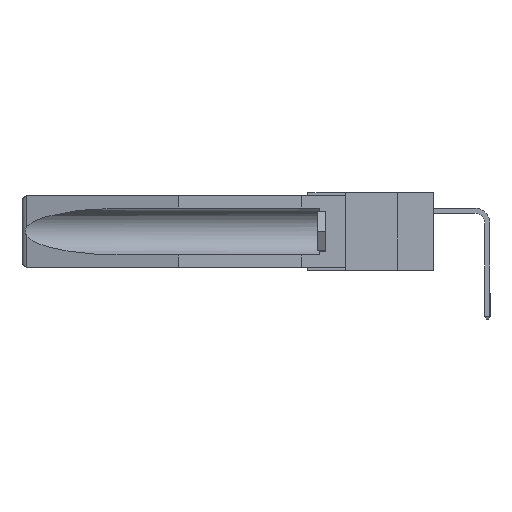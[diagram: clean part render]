
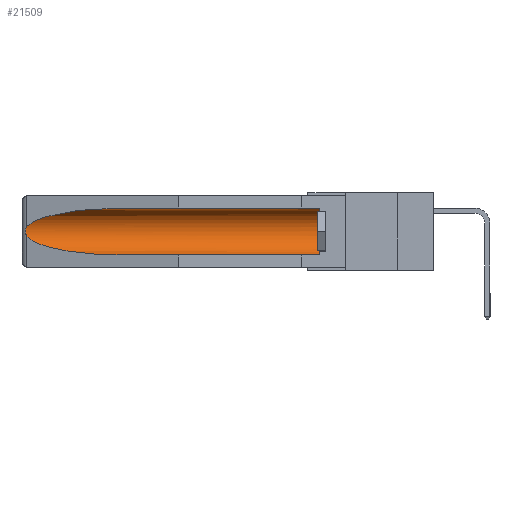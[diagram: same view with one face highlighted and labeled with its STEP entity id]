
A CAD part, left-side view. The second image highlights one B-rep face of the part: STEP entity #21509.
In plain terms, the highlighted cylindrical face has radius 2.857 mm (diameter 5.715 mm), a partial arc.
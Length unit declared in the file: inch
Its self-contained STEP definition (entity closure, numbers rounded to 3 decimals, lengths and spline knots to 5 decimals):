
#577 = CARTESIAN_POINT ( 'NONE',  ( 0.155, 0.126, -0.059 ) ) ;
#893 = DIRECTION ( 'NONE',  ( 0., -1., 0. ) ) ;
#1407 = VECTOR ( 'NONE', #24017, 39.37008 ) ;
#2414 = CARTESIAN_POINT ( 'NONE',  ( 0.26537, 1.52718, -0.14972 ) ) ;
#2586 = CYLINDRICAL_SURFACE ( 'NONE', #2621, 0.1125 ) ;
#2621 = AXIS2_PLACEMENT_3D ( 'NONE', #10202, #10101, #19785 ) ;
#2776 = ORIENTED_EDGE ( 'NONE', *, *, #7997, .T. ) ;
#2848 = CARTESIAN_POINT ( 'NONE',  ( 0.2673, 1.5327, -0.16383 ) ) ;
#3377 = FACE_OUTER_BOUND ( 'NONE', #18006, .T. ) ;
#3425 = CARTESIAN_POINT ( 'NONE',  ( 0.155, 1.07973, -0.059 ) ) ;
#3851 = EDGE_CURVE ( 'NONE', #27591, #8074, #8372, .T. ) ;
#4380 =( BOUNDED_CURVE ( )  B_SPLINE_CURVE ( 3, ( #20080, #9997, #12568, #12456 ),
 .UNSPECIFIED., .F., .F. ) 
 B_SPLINE_CURVE_WITH_KNOTS ( ( 4, 4 ),
 ( 0.1948, 1.5708 ),
 .UNSPECIFIED. ) 
 CURVE ( )  GEOMETRIC_REPRESENTATION_ITEM ( )  RATIONAL_B_SPLINE_CURVE ( ( 1., 0.848, 0.848, 1. ) ) 
 REPRESENTATION_ITEM ( '' )  );
#4825 = VERTEX_POINT ( 'NONE', #29679 ) ;
#4939 = CARTESIAN_POINT ( 'NONE',  ( 0.2675, 1.53308, -0.16763 ) ) ;
#5349 = CARTESIAN_POINT ( 'NONE',  ( 0.26654, 1.53092, -0.15636 ) ) ;
#5890 = DIRECTION ( 'NONE',  ( 0., 0., 1. ) ) ;
#6041 = CARTESIAN_POINT ( 'NONE',  ( 0.155, 0.126, -0.284 ) ) ;
#6759 = B_SPLINE_CURVE_WITH_KNOTS ( 'NONE', 3,
 ( #2414, #20089, #5349, #2848, #4939, #22578, #27215, #12468, #12373, #25037 ),
 .UNSPECIFIED., .F., .F.,
 ( 4, 2, 2, 2, 4 ),
 ( 0., 0.00029, 0.00058, 0.00087, 0.00117 ),
 .UNSPECIFIED. ) ;
#7787 = CARTESIAN_POINT ( 'NONE',  ( 0.26537, 1.52718, -0.19328 ) ) ;
#7997 = EDGE_CURVE ( 'NONE', #20278, #27591, #26233, .T. ) ;
#8074 = VERTEX_POINT ( 'NONE', #3425 ) ;
#8372 = LINE ( 'NONE', #26390, #1407 ) ;
#8554 =( BOUNDED_CURVE ( )  B_SPLINE_CURVE ( 3, ( #27789, #20243, #15435, #24977 ),
 .UNSPECIFIED., .F., .F. ) 
 B_SPLINE_CURVE_WITH_KNOTS ( ( 4, 4 ),
 ( 4.71239, 6.08839 ),
 .UNSPECIFIED. ) 
 CURVE ( )  GEOMETRIC_REPRESENTATION_ITEM ( )  RATIONAL_B_SPLINE_CURVE ( ( 1., 0.848, 0.848, 1. ) ) 
 REPRESENTATION_ITEM ( '' )  );
#8828 = VECTOR ( 'NONE', #14653, 39.37008 ) ;
#9297 = EDGE_CURVE ( 'NONE', #20278, #16588, #30841, .T. ) ;
#9997 = CARTESIAN_POINT ( 'NONE',  ( 0.25451, 1.48313, -0.24835 ) ) ;
#10101 = DIRECTION ( 'NONE',  ( 0., 1., 0. ) ) ;
#10202 = CARTESIAN_POINT ( 'NONE',  ( 0.155, -0.30754, -0.1715 ) ) ;
#10819 = EDGE_CURVE ( 'NONE', #8074, #4825, #8554, .T. ) ;
#11941 = EDGE_CURVE ( 'NONE', #15823, #16588, #4380, .T. ) ;
#12373 = CARTESIAN_POINT ( 'NONE',  ( 0.26597, 1.5296, -0.19026 ) ) ;
#12456 = CARTESIAN_POINT ( 'NONE',  ( 0.155, 1.07973, -0.284 ) ) ;
#12468 = CARTESIAN_POINT ( 'NONE',  ( 0.26655, 1.53094, -0.18657 ) ) ;
#12568 = CARTESIAN_POINT ( 'NONE',  ( 0.21114, 1.30732, -0.284 ) ) ;
#13247 = CARTESIAN_POINT ( 'NONE',  ( 0.155, 0.126, -0.1715 ) ) ;
#14653 = DIRECTION ( 'NONE',  ( 0., 1., 0. ) ) ;
#15435 = CARTESIAN_POINT ( 'NONE',  ( 0.25451, 1.48313, -0.09465 ) ) ;
#15823 = VERTEX_POINT ( 'NONE', #7787 ) ;
#16588 = VERTEX_POINT ( 'NONE', #21506 ) ;
#17845 = ORIENTED_EDGE ( 'NONE', *, *, #3851, .T. ) ;
#18006 = EDGE_LOOP ( 'NONE', ( #25649, #25445, #29173, #28825, #2776, #17845 ) ) ;
#19785 = DIRECTION ( 'NONE',  ( 0., 0., 1. ) ) ;
#20080 = CARTESIAN_POINT ( 'NONE',  ( 0.26537, 1.52718, -0.19328 ) ) ;
#20089 = CARTESIAN_POINT ( 'NONE',  ( 0.26597, 1.52961, -0.15275 ) ) ;
#20243 = CARTESIAN_POINT ( 'NONE',  ( 0.21114, 1.30732, -0.059 ) ) ;
#20278 = VERTEX_POINT ( 'NONE', #6041 ) ;
#21506 = CARTESIAN_POINT ( 'NONE',  ( 0.155, 1.07973, -0.284 ) ) ;
#21509 = ADVANCED_FACE ( 'NONE', ( #3377 ), #2586, .F. ) ;
#22139 = CARTESIAN_POINT ( 'NONE',  ( 0.155, -0.30754, -0.284 ) ) ;
#22502 = EDGE_CURVE ( 'NONE', #4825, #15823, #6759, .T. ) ;
#22578 = CARTESIAN_POINT ( 'NONE',  ( 0.2675, 1.53308, -0.17534 ) ) ;
#24017 = DIRECTION ( 'NONE',  ( 0., 1., 0. ) ) ;
#24977 = CARTESIAN_POINT ( 'NONE',  ( 0.26537, 1.52718, -0.14972 ) ) ;
#25037 = CARTESIAN_POINT ( 'NONE',  ( 0.26537, 1.52718, -0.19328 ) ) ;
#25445 = ORIENTED_EDGE ( 'NONE', *, *, #22502, .T. ) ;
#25649 = ORIENTED_EDGE ( 'NONE', *, *, #10819, .T. ) ;
#26233 = CIRCLE ( 'NONE', #26742, 0.1125 ) ;
#26390 = CARTESIAN_POINT ( 'NONE',  ( 0.155, -0.30754, -0.059 ) ) ;
#26742 = AXIS2_PLACEMENT_3D ( 'NONE', #13247, #893, #5890 ) ;
#27215 = CARTESIAN_POINT ( 'NONE',  ( 0.2673, 1.53269, -0.17917 ) ) ;
#27591 = VERTEX_POINT ( 'NONE', #577 ) ;
#27789 = CARTESIAN_POINT ( 'NONE',  ( 0.155, 1.07973, -0.059 ) ) ;
#28825 = ORIENTED_EDGE ( 'NONE', *, *, #9297, .F. ) ;
#29173 = ORIENTED_EDGE ( 'NONE', *, *, #11941, .T. ) ;
#29679 = CARTESIAN_POINT ( 'NONE',  ( 0.26537, 1.52718, -0.14972 ) ) ;
#30841 = LINE ( 'NONE', #22139, #8828 ) ;
